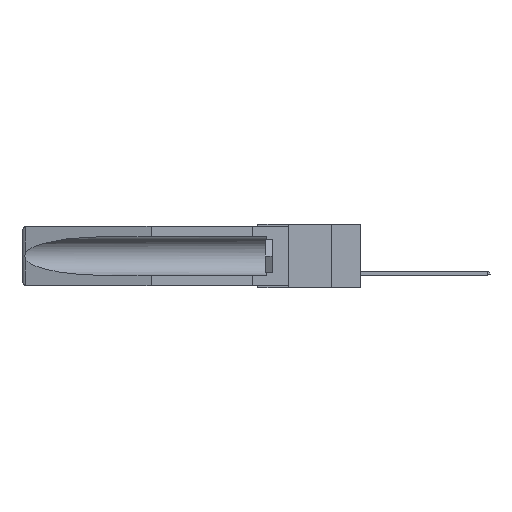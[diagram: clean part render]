
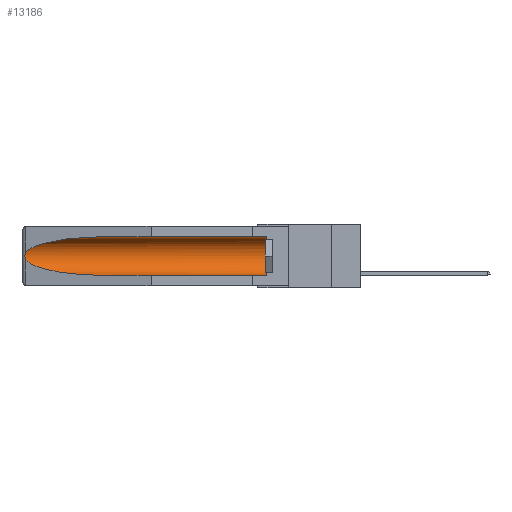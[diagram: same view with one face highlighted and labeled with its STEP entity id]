
A CAD part, left-side view. The second image highlights one B-rep face of the part: STEP entity #13186.
In plain terms, the highlighted cylindrical face has radius 2.857 mm (diameter 5.715 mm), a partial arc.
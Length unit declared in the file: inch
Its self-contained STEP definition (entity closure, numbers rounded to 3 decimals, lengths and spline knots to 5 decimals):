
#261 = B_SPLINE_CURVE_WITH_KNOTS ( 'NONE', 3,
 ( #17972, #2479, #6167, #2402, #20064, #16352, #12169, #24009, #10257, #4281 ),
 .UNSPECIFIED., .F., .F.,
 ( 4, 2, 2, 2, 4 ),
 ( 0., 0.00029, 0.00058, 0.00087, 0.00117 ),
 .UNSPECIFIED. ) ;
#638 = AXIS2_PLACEMENT_3D ( 'NONE', #4813, #20769, #10806 ) ;
#1235 = ORIENTED_EDGE ( 'NONE', *, *, #4737, .T. ) ;
#1307 = CIRCLE ( 'NONE', #22874, 0.1125 ) ;
#1460 = DIRECTION ( 'NONE',  ( 0., 1., 0. ) ) ;
#1479 = ORIENTED_EDGE ( 'NONE', *, *, #24292, .T. ) ;
#1551 = CARTESIAN_POINT ( 'NONE',  ( 0.155, -0.30754, -0.284 ) ) ;
#1592 = CARTESIAN_POINT ( 'NONE',  ( 0.155, 1.07973, -0.284 ) ) ;
#1766 = CARTESIAN_POINT ( 'NONE',  ( 0.155, -0.30754, -0.059 ) ) ;
#2014 = VECTOR ( 'NONE', #4039, 39.37008 ) ;
#2402 = CARTESIAN_POINT ( 'NONE',  ( 0.2673, 1.5327, -0.16383 ) ) ;
#2479 = CARTESIAN_POINT ( 'NONE',  ( 0.26597, 1.52961, -0.15275 ) ) ;
#2697 = ORIENTED_EDGE ( 'NONE', *, *, #23707, .F. ) ;
#3233 = EDGE_CURVE ( 'NONE', #15549, #14257, #261, .T. ) ;
#3740 =( BOUNDED_CURVE ( )  B_SPLINE_CURVE ( 3, ( #18285, #6491, #6317, #22265 ),
 .UNSPECIFIED., .F., .F. ) 
 B_SPLINE_CURVE_WITH_KNOTS ( ( 4, 4 ),
 ( 0.1948, 1.5708 ),
 .UNSPECIFIED. ) 
 CURVE ( )  GEOMETRIC_REPRESENTATION_ITEM ( )  RATIONAL_B_SPLINE_CURVE ( ( 1., 0.848, 0.848, 1. ) ) 
 REPRESENTATION_ITEM ( '' )  );
#4039 = DIRECTION ( 'NONE',  ( 0., 1., 0. ) ) ;
#4281 = CARTESIAN_POINT ( 'NONE',  ( 0.26537, 1.52718, -0.19328 ) ) ;
#4737 = EDGE_CURVE ( 'NONE', #14257, #7395, #3740, .T. ) ;
#4738 = CARTESIAN_POINT ( 'NONE',  ( 0.155, 0.126, -0.1715 ) ) ;
#4813 = CARTESIAN_POINT ( 'NONE',  ( 0.155, -0.30754, -0.1715 ) ) ;
#5041 = CARTESIAN_POINT ( 'NONE',  ( 0.155, 1.07973, -0.059 ) ) ;
#5343 = ORIENTED_EDGE ( 'NONE', *, *, #18305, .T. ) ;
#6167 = CARTESIAN_POINT ( 'NONE',  ( 0.26654, 1.53092, -0.15636 ) ) ;
#6317 = CARTESIAN_POINT ( 'NONE',  ( 0.21114, 1.30732, -0.284 ) ) ;
#6402 = DIRECTION ( 'NONE',  ( 0., -1., 0. ) ) ;
#6491 = CARTESIAN_POINT ( 'NONE',  ( 0.25451, 1.48313, -0.24835 ) ) ;
#6812 = VERTEX_POINT ( 'NONE', #5041 ) ;
#7117 = EDGE_CURVE ( 'NONE', #20882, #11483, #1307, .T. ) ;
#7395 = VERTEX_POINT ( 'NONE', #1592 ) ;
#7633 = CARTESIAN_POINT ( 'NONE',  ( 0.26537, 1.52718, -0.19328 ) ) ;
#9426 = LINE ( 'NONE', #1766, #2014 ) ;
#9715 = CARTESIAN_POINT ( 'NONE',  ( 0.155, 0.126, -0.059 ) ) ;
#10247 = ORIENTED_EDGE ( 'NONE', *, *, #7117, .T. ) ;
#10257 = CARTESIAN_POINT ( 'NONE',  ( 0.26597, 1.5296, -0.19026 ) ) ;
#10649 = LINE ( 'NONE', #1551, #16233 ) ;
#10806 = DIRECTION ( 'NONE',  ( 0., 0., 1. ) ) ;
#11483 = VERTEX_POINT ( 'NONE', #9715 ) ;
#12169 = CARTESIAN_POINT ( 'NONE',  ( 0.2673, 1.53269, -0.17917 ) ) ;
#13186 = ADVANCED_FACE ( 'NONE', ( #21401 ), #20148, .F. ) ;
#14257 = VERTEX_POINT ( 'NONE', #7633 ) ;
#15503 = CARTESIAN_POINT ( 'NONE',  ( 0.25451, 1.48313, -0.09465 ) ) ;
#15549 = VERTEX_POINT ( 'NONE', #17166 ) ;
#16233 = VECTOR ( 'NONE', #1460, 39.37008 ) ;
#16352 = CARTESIAN_POINT ( 'NONE',  ( 0.2675, 1.53308, -0.17534 ) ) ;
#17166 = CARTESIAN_POINT ( 'NONE',  ( 0.26537, 1.52718, -0.14972 ) ) ;
#17184 = ORIENTED_EDGE ( 'NONE', *, *, #3233, .T. ) ;
#17566 = CARTESIAN_POINT ( 'NONE',  ( 0.21114, 1.30732, -0.059 ) ) ;
#17972 = CARTESIAN_POINT ( 'NONE',  ( 0.26537, 1.52718, -0.14972 ) ) ;
#18285 = CARTESIAN_POINT ( 'NONE',  ( 0.26537, 1.52718, -0.19328 ) ) ;
#18305 = EDGE_CURVE ( 'NONE', #11483, #6812, #9426, .T. ) ;
#18449 = DIRECTION ( 'NONE',  ( 0., 0., 1. ) ) ;
#19382 = CARTESIAN_POINT ( 'NONE',  ( 0.155, 1.07973, -0.059 ) ) ;
#19473 = CARTESIAN_POINT ( 'NONE',  ( 0.26537, 1.52718, -0.14972 ) ) ;
#20064 = CARTESIAN_POINT ( 'NONE',  ( 0.2675, 1.53308, -0.16763 ) ) ;
#20148 = CYLINDRICAL_SURFACE ( 'NONE', #638, 0.1125 ) ;
#20769 = DIRECTION ( 'NONE',  ( 0., 1., 0. ) ) ;
#20882 = VERTEX_POINT ( 'NONE', #25071 ) ;
#21054 =( BOUNDED_CURVE ( )  B_SPLINE_CURVE ( 3, ( #19382, #17566, #15503, #19473 ),
 .UNSPECIFIED., .F., .F. ) 
 B_SPLINE_CURVE_WITH_KNOTS ( ( 4, 4 ),
 ( 4.71239, 6.08839 ),
 .UNSPECIFIED. ) 
 CURVE ( )  GEOMETRIC_REPRESENTATION_ITEM ( )  RATIONAL_B_SPLINE_CURVE ( ( 1., 0.848, 0.848, 1. ) ) 
 REPRESENTATION_ITEM ( '' )  );
#21401 = FACE_OUTER_BOUND ( 'NONE', #23415, .T. ) ;
#22265 = CARTESIAN_POINT ( 'NONE',  ( 0.155, 1.07973, -0.284 ) ) ;
#22874 = AXIS2_PLACEMENT_3D ( 'NONE', #4738, #6402, #18449 ) ;
#23415 = EDGE_LOOP ( 'NONE', ( #1479, #17184, #1235, #2697, #10247, #5343 ) ) ;
#23707 = EDGE_CURVE ( 'NONE', #20882, #7395, #10649, .T. ) ;
#24009 = CARTESIAN_POINT ( 'NONE',  ( 0.26655, 1.53094, -0.18657 ) ) ;
#24292 = EDGE_CURVE ( 'NONE', #6812, #15549, #21054, .T. ) ;
#25071 = CARTESIAN_POINT ( 'NONE',  ( 0.155, 0.126, -0.284 ) ) ;
